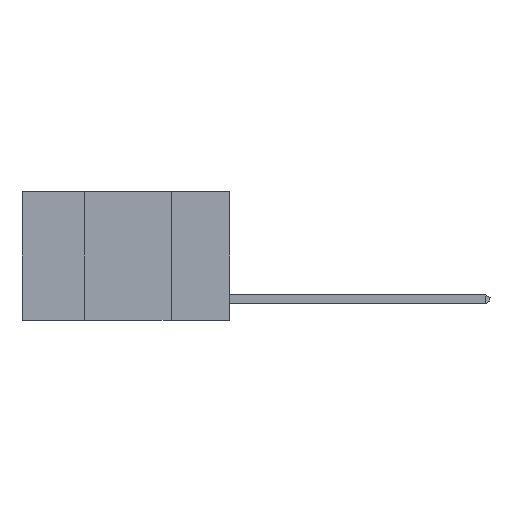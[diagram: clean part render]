
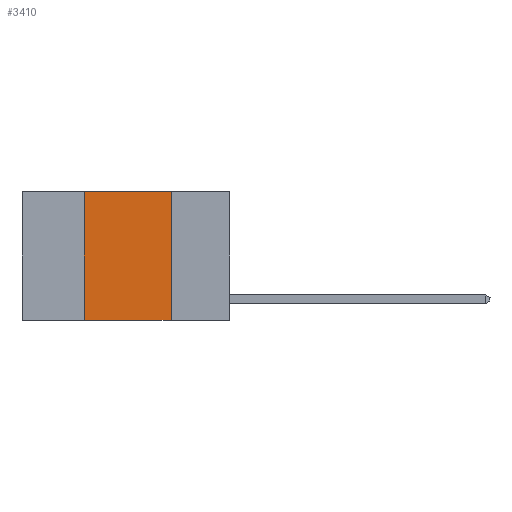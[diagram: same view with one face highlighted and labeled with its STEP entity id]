
A CAD part, left-side view. The second image highlights one B-rep face of the part: STEP entity #3410.
In plain terms, the highlighted planar face has unit normal (-1, 0, 0).
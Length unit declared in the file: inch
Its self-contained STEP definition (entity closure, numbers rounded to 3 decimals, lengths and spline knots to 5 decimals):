
#633 = DIRECTION ( 'NONE',  ( 0., 0., -1. ) ) ;
#3410 = ADVANCED_FACE ( 'NONE', ( #21170 ), #9962, .F. ) ;
#4401 = VERTEX_POINT ( 'NONE', #13035 ) ;
#4983 = CARTESIAN_POINT ( 'NONE',  ( 0., 0.6, 0. ) ) ;
#5463 = EDGE_CURVE ( 'NONE', #28168, #4401, #20459, .T. ) ;
#5743 = CARTESIAN_POINT ( 'NONE',  ( 0., 0.42, 0. ) ) ;
#6552 = ORIENTED_EDGE ( 'NONE', *, *, #17077, .F. ) ;
#6840 = VECTOR ( 'NONE', #15373, 39.37008 ) ;
#6980 = CARTESIAN_POINT ( 'NONE',  ( 0., 0.42, 0. ) ) ;
#7300 = VECTOR ( 'NONE', #633, 39.37008 ) ;
#7449 = CARTESIAN_POINT ( 'NONE',  ( 0., 0.6, 0. ) ) ;
#7831 = DIRECTION ( 'NONE',  ( 0., -1., 0. ) ) ;
#8039 = VECTOR ( 'NONE', #7831, 39.37008 ) ;
#8594 = VECTOR ( 'NONE', #16008, 39.37008 ) ;
#9962 = PLANE ( 'NONE',  #26748 ) ;
#10192 = LINE ( 'NONE', #16398, #8039 ) ;
#10819 = LINE ( 'NONE', #6980, #6840 ) ;
#11511 = CARTESIAN_POINT ( 'NONE',  ( 0., 0.17, 0. ) ) ;
#11796 = LINE ( 'NONE', #11511, #7300 ) ;
#13035 = CARTESIAN_POINT ( 'NONE',  ( 0., 0.17, 0. ) ) ;
#13990 = CARTESIAN_POINT ( 'NONE',  ( 0., 0.42, -0.37 ) ) ;
#15373 = DIRECTION ( 'NONE',  ( 0., 0., 1. ) ) ;
#16008 = DIRECTION ( 'NONE',  ( 0., -1., 0. ) ) ;
#16398 = CARTESIAN_POINT ( 'NONE',  ( 0., 0.6, -0.37 ) ) ;
#16740 = DIRECTION ( 'NONE',  ( 0., 0., -1. ) ) ;
#17077 = EDGE_CURVE ( 'NONE', #22929, #28168, #10819, .T. ) ;
#17612 = EDGE_CURVE ( 'NONE', #4401, #18729, #11796, .T. ) ;
#18194 = CARTESIAN_POINT ( 'NONE',  ( 0., 0.17, -0.37 ) ) ;
#18729 = VERTEX_POINT ( 'NONE', #18194 ) ;
#18971 = DIRECTION ( 'NONE',  ( 1., 0., 0. ) ) ;
#19102 = EDGE_LOOP ( 'NONE', ( #27786, #19787, #6552, #24202 ) ) ;
#19787 = ORIENTED_EDGE ( 'NONE', *, *, #5463, .F. ) ;
#20459 = LINE ( 'NONE', #7449, #8594 ) ;
#21170 = FACE_OUTER_BOUND ( 'NONE', #19102, .T. ) ;
#22450 = EDGE_CURVE ( 'NONE', #22929, #18729, #10192, .T. ) ;
#22929 = VERTEX_POINT ( 'NONE', #13990 ) ;
#24202 = ORIENTED_EDGE ( 'NONE', *, *, #22450, .T. ) ;
#26748 = AXIS2_PLACEMENT_3D ( 'NONE', #4983, #18971, #16740 ) ;
#27786 = ORIENTED_EDGE ( 'NONE', *, *, #17612, .F. ) ;
#28168 = VERTEX_POINT ( 'NONE', #5743 ) ;
